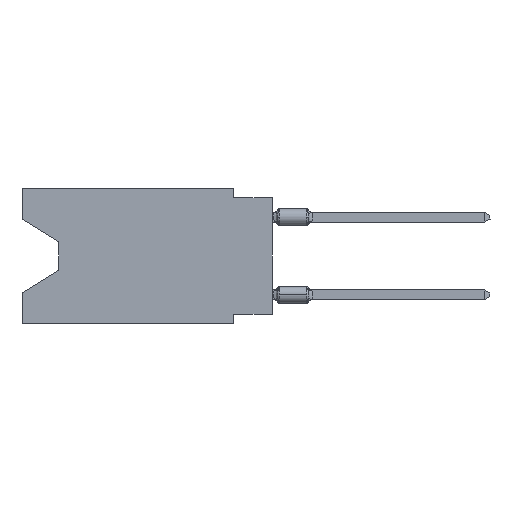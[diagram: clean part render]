
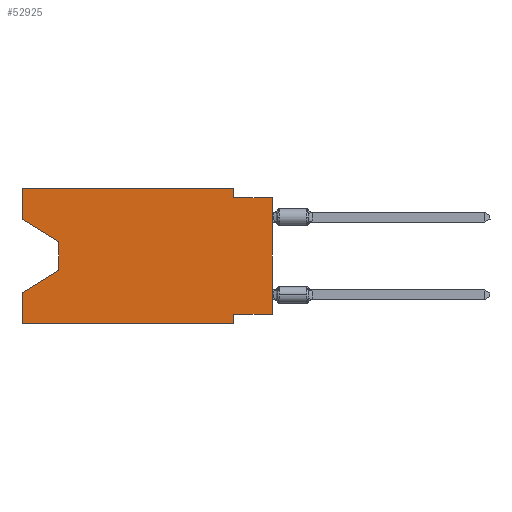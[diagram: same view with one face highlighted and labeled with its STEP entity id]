
A CAD part, left-side view. The second image highlights one B-rep face of the part: STEP entity #52925.
In plain terms, the highlighted planar face has unit normal (-1, 0, 0).
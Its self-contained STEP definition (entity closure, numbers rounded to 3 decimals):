
#2 = VECTOR ( 'NONE', #12091, 1000. ) ;
#457 = LINE ( 'NONE', #51449, #36910 ) ;
#945 = CARTESIAN_POINT ( 'NONE',  ( 0., 16.383, -2.038 ) ) ;
#2615 = EDGE_CURVE ( 'NONE', #43811, #40686, #50263, .T. ) ;
#3154 = VERTEX_POINT ( 'NONE', #43856 ) ;
#4086 = ORIENTED_EDGE ( 'NONE', *, *, #56582, .F. ) ;
#5421 = CARTESIAN_POINT ( 'NONE',  ( 0., 16.383, -2.038 ) ) ;
#5597 = VERTEX_POINT ( 'NONE', #31821 ) ;
#6809 = ORIENTED_EDGE ( 'NONE', *, *, #13681, .T. ) ;
#7110 = DIRECTION ( 'NONE',  ( 0., 0., 1. ) ) ;
#8771 = CARTESIAN_POINT ( 'NONE',  ( 0., 16.383, 0. ) ) ;
#9017 = ORIENTED_EDGE ( 'NONE', *, *, #45837, .F. ) ;
#9227 = VECTOR ( 'NONE', #61024, 1000. ) ;
#9699 = LINE ( 'NONE', #8771, #28947 ) ;
#12091 = DIRECTION ( 'NONE',  ( 0., -1., 0. ) ) ;
#12220 = CARTESIAN_POINT ( 'NONE',  ( 0., 2.54, -8.89 ) ) ;
#12841 = LINE ( 'NONE', #60710, #9227 ) ;
#12887 = CARTESIAN_POINT ( 'NONE',  ( 0., 13.97, -5.385 ) ) ;
#13681 = EDGE_CURVE ( 'NONE', #3154, #40686, #12841, .T. ) ;
#14049 = ORIENTED_EDGE ( 'NONE', *, *, #44990, .T. ) ;
#14116 = DIRECTION ( 'NONE',  ( 0., 0., -1. ) ) ;
#15626 = VECTOR ( 'NONE', #26646, 1000. ) ;
#16135 = LINE ( 'NONE', #20200, #44541 ) ;
#17643 = DIRECTION ( 'NONE',  ( 0., 0.855, -0.519 ) ) ;
#17936 = EDGE_CURVE ( 'NONE', #36254, #43811, #43908, .T. ) ;
#18043 = VERTEX_POINT ( 'NONE', #50097 ) ;
#18474 = EDGE_LOOP ( 'NONE', ( #55852, #48089, #14049, #33425, #51169, #32081, #9017, #6809, #38060, #37209, #21893, #4086 ) ) ;
#19706 = LINE ( 'NONE', #56721, #54790 ) ;
#19908 = DIRECTION ( 'NONE',  ( 0., -0.855, -0.519 ) ) ;
#20200 = CARTESIAN_POINT ( 'NONE',  ( 0., 13.97, -3.505 ) ) ;
#20583 = CARTESIAN_POINT ( 'NONE',  ( 0., 2.54, 0. ) ) ;
#21893 = ORIENTED_EDGE ( 'NONE', *, *, #57238, .F. ) ;
#22458 = EDGE_CURVE ( 'NONE', #18043, #36212, #49710, .T. ) ;
#22536 = VERTEX_POINT ( 'NONE', #42220 ) ;
#24394 = DIRECTION ( 'NONE',  ( 0., -1., 0. ) ) ;
#26001 = CARTESIAN_POINT ( 'NONE',  ( 0., 13.97, -3.505 ) ) ;
#26089 = CARTESIAN_POINT ( 'NONE',  ( 0., 16.383, -8.89 ) ) ;
#26435 = VECTOR ( 'NONE', #19908, 1000. ) ;
#26646 = DIRECTION ( 'NONE',  ( 0., -1., 0. ) ) ;
#27278 = CARTESIAN_POINT ( 'NONE',  ( 0., 2.54, -0.635 ) ) ;
#27437 = CARTESIAN_POINT ( 'NONE',  ( 0., 2.54, 0. ) ) ;
#27710 = VERTEX_POINT ( 'NONE', #46247 ) ;
#27738 = DIRECTION ( 'NONE',  ( 0., 0., 1. ) ) ;
#28947 = VECTOR ( 'NONE', #27738, 1000. ) ;
#31795 = CARTESIAN_POINT ( 'NONE',  ( 0., 0., -8.255 ) ) ;
#31821 = CARTESIAN_POINT ( 'NONE',  ( 0., 16.383, 0. ) ) ;
#32081 = ORIENTED_EDGE ( 'NONE', *, *, #34712, .F. ) ;
#33425 = ORIENTED_EDGE ( 'NONE', *, *, #44192, .F. ) ;
#34712 = EDGE_CURVE ( 'NONE', #22536, #36212, #19706, .T. ) ;
#34780 = VERTEX_POINT ( 'NONE', #5421 ) ;
#35110 = DIRECTION ( 'NONE',  ( 0., 0., -1. ) ) ;
#36212 = VERTEX_POINT ( 'NONE', #12220 ) ;
#36254 = VERTEX_POINT ( 'NONE', #27437 ) ;
#36910 = VECTOR ( 'NONE', #24394, 1000. ) ;
#37209 = ORIENTED_EDGE ( 'NONE', *, *, #17936, .F. ) ;
#38060 = ORIENTED_EDGE ( 'NONE', *, *, #2615, .F. ) ;
#38678 = VERTEX_POINT ( 'NONE', #12887 ) ;
#39430 = VECTOR ( 'NONE', #44518, 1000. ) ;
#39787 = LINE ( 'NONE', #945, #26435 ) ;
#40428 = CARTESIAN_POINT ( 'NONE',  ( 0., 0., -0.635 ) ) ;
#40686 = VERTEX_POINT ( 'NONE', #40428 ) ;
#41300 = CARTESIAN_POINT ( 'NONE',  ( 0., 16.383, 0. ) ) ;
#41881 = CARTESIAN_POINT ( 'NONE',  ( 0., 13.97, -5.385 ) ) ;
#42220 = CARTESIAN_POINT ( 'NONE',  ( 0., 2.54, -8.255 ) ) ;
#43811 = VERTEX_POINT ( 'NONE', #27278 ) ;
#43856 = CARTESIAN_POINT ( 'NONE',  ( 0., 0., -8.255 ) ) ;
#43908 = LINE ( 'NONE', #20583, #39430 ) ;
#44192 = EDGE_CURVE ( 'NONE', #18043, #27710, #9699, .T. ) ;
#44428 = CARTESIAN_POINT ( 'NONE',  ( 0., 16.383, 0. ) ) ;
#44518 = DIRECTION ( 'NONE',  ( 0., 0., -1. ) ) ;
#44541 = VECTOR ( 'NONE', #35110, 1000. ) ;
#44990 = EDGE_CURVE ( 'NONE', #38678, #27710, #51526, .T. ) ;
#45059 = DIRECTION ( 'NONE',  ( 1., 0., 0. ) ) ;
#45367 = PLANE ( 'NONE',  #56517 ) ;
#45837 = EDGE_CURVE ( 'NONE', #3154, #22536, #55424, .T. ) ;
#45912 = VECTOR ( 'NONE', #17643, 1000. ) ;
#46247 = CARTESIAN_POINT ( 'NONE',  ( 0., 16.383, -6.852 ) ) ;
#46414 = VERTEX_POINT ( 'NONE', #26001 ) ;
#48089 = ORIENTED_EDGE ( 'NONE', *, *, #51519, .T. ) ;
#49376 = EDGE_CURVE ( 'NONE', #34780, #46414, #39787, .T. ) ;
#49710 = LINE ( 'NONE', #26089, #2 ) ;
#49961 = CARTESIAN_POINT ( 'NONE',  ( 0., 0., -0.635 ) ) ;
#50030 = FACE_OUTER_BOUND ( 'NONE', #18474, .T. ) ;
#50097 = CARTESIAN_POINT ( 'NONE',  ( 0., 16.383, -8.89 ) ) ;
#50263 = LINE ( 'NONE', #49961, #15626 ) ;
#50757 = DIRECTION ( 'NONE',  ( 0., 1., 0. ) ) ;
#50900 = VECTOR ( 'NONE', #50757, 1000. ) ;
#51169 = ORIENTED_EDGE ( 'NONE', *, *, #22458, .T. ) ;
#51449 = CARTESIAN_POINT ( 'NONE',  ( 0., 16.383, 0. ) ) ;
#51519 = EDGE_CURVE ( 'NONE', #46414, #38678, #16135, .T. ) ;
#51526 = LINE ( 'NONE', #41881, #45912 ) ;
#52925 = ADVANCED_FACE ( 'NONE', ( #50030 ), #45367, .F. ) ;
#54790 = VECTOR ( 'NONE', #14116, 1000. ) ;
#55424 = LINE ( 'NONE', #31795, #50900 ) ;
#55852 = ORIENTED_EDGE ( 'NONE', *, *, #49376, .T. ) ;
#56517 = AXIS2_PLACEMENT_3D ( 'NONE', #41300, #45059, #60263 ) ;
#56582 = EDGE_CURVE ( 'NONE', #34780, #5597, #58108, .T. ) ;
#56721 = CARTESIAN_POINT ( 'NONE',  ( 0., 2.54, -8.89 ) ) ;
#57238 = EDGE_CURVE ( 'NONE', #5597, #36254, #457, .T. ) ;
#58108 = LINE ( 'NONE', #44428, #60613 ) ;
#60263 = DIRECTION ( 'NONE',  ( 0., 0., -1. ) ) ;
#60613 = VECTOR ( 'NONE', #7110, 1000. ) ;
#60710 = CARTESIAN_POINT ( 'NONE',  ( 0., 0., 0. ) ) ;
#61024 = DIRECTION ( 'NONE',  ( 0., 0., 1. ) ) ;
